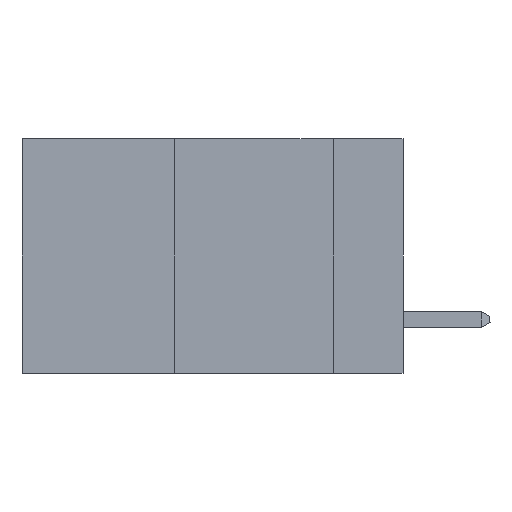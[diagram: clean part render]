
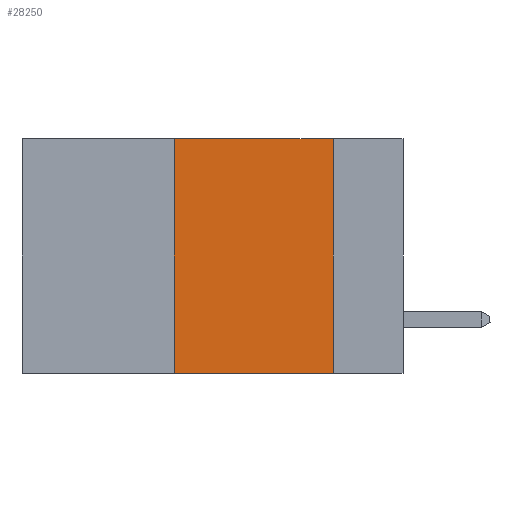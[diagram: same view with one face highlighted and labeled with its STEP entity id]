
A CAD part, left-side view. The second image highlights one B-rep face of the part: STEP entity #28250.
In plain terms, the highlighted planar face has unit normal (-1, 0, 0).
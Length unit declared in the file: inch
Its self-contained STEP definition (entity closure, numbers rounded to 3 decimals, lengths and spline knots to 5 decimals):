
#337 = DIRECTION ( 'NONE',  ( 0., 0., -1. ) ) ;
#707 = DIRECTION ( 'NONE',  ( 0., -1., 0. ) ) ;
#1010 = ORIENTED_EDGE ( 'NONE', *, *, #21402, .F. ) ;
#2551 = ORIENTED_EDGE ( 'NONE', *, *, #13515, .F. ) ;
#2601 = CARTESIAN_POINT ( 'NONE',  ( 0., 0.36, -0.37 ) ) ;
#4059 = LINE ( 'NONE', #15132, #16765 ) ;
#4845 = DIRECTION ( 'NONE',  ( 0., -1., 0. ) ) ;
#7109 = CARTESIAN_POINT ( 'NONE',  ( 0., 0.36, 0. ) ) ;
#7255 = VECTOR ( 'NONE', #4845, 39.37008 ) ;
#10307 = LINE ( 'NONE', #15083, #28717 ) ;
#11337 = CARTESIAN_POINT ( 'NONE',  ( 0., 0.6, 0. ) ) ;
#11542 = EDGE_CURVE ( 'NONE', #31110, #20761, #10307, .T. ) ;
#11743 = PLANE ( 'NONE',  #30056 ) ;
#12408 = DIRECTION ( 'NONE',  ( 0., 0., 1. ) ) ;
#12541 = VERTEX_POINT ( 'NONE', #7109 ) ;
#13515 = EDGE_CURVE ( 'NONE', #31110, #12541, #4059, .T. ) ;
#14001 = VECTOR ( 'NONE', #337, 39.37008 ) ;
#14158 = DIRECTION ( 'NONE',  ( 0., 0., -1. ) ) ;
#14207 = CARTESIAN_POINT ( 'NONE',  ( 0., 0.6, 0. ) ) ;
#15083 = CARTESIAN_POINT ( 'NONE',  ( 0., 0.6, -0.37 ) ) ;
#15132 = CARTESIAN_POINT ( 'NONE',  ( 0., 0.36, 0. ) ) ;
#15340 = VERTEX_POINT ( 'NONE', #28336 ) ;
#15796 = EDGE_CURVE ( 'NONE', #12541, #15340, #28294, .T. ) ;
#16157 = ORIENTED_EDGE ( 'NONE', *, *, #11542, .T. ) ;
#16230 = EDGE_LOOP ( 'NONE', ( #1010, #25344, #2551, #16157 ) ) ;
#16765 = VECTOR ( 'NONE', #12408, 39.37008 ) ;
#18870 = LINE ( 'NONE', #29012, #14001 ) ;
#20761 = VERTEX_POINT ( 'NONE', #21568 ) ;
#21402 = EDGE_CURVE ( 'NONE', #15340, #20761, #18870, .T. ) ;
#21568 = CARTESIAN_POINT ( 'NONE',  ( 0., 0.11, -0.37 ) ) ;
#22385 = FACE_OUTER_BOUND ( 'NONE', #16230, .T. ) ;
#25344 = ORIENTED_EDGE ( 'NONE', *, *, #15796, .F. ) ;
#28250 = ADVANCED_FACE ( 'NONE', ( #22385 ), #11743, .F. ) ;
#28294 = LINE ( 'NONE', #14207, #7255 ) ;
#28336 = CARTESIAN_POINT ( 'NONE',  ( 0., 0.11, 0. ) ) ;
#28499 = DIRECTION ( 'NONE',  ( 1., 0., 0. ) ) ;
#28717 = VECTOR ( 'NONE', #707, 39.37008 ) ;
#29012 = CARTESIAN_POINT ( 'NONE',  ( 0., 0.11, 0. ) ) ;
#30056 = AXIS2_PLACEMENT_3D ( 'NONE', #11337, #28499, #14158 ) ;
#31110 = VERTEX_POINT ( 'NONE', #2601 ) ;
